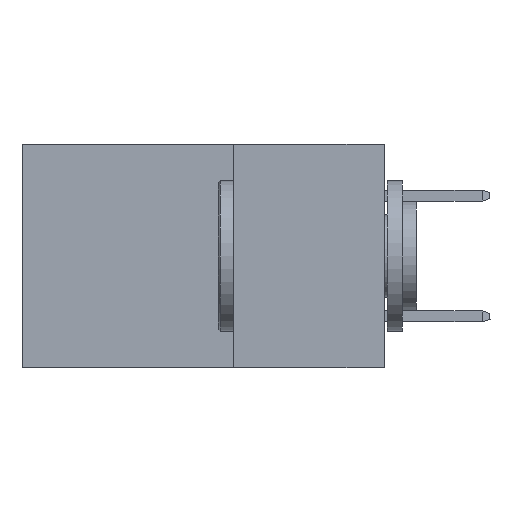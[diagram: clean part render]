
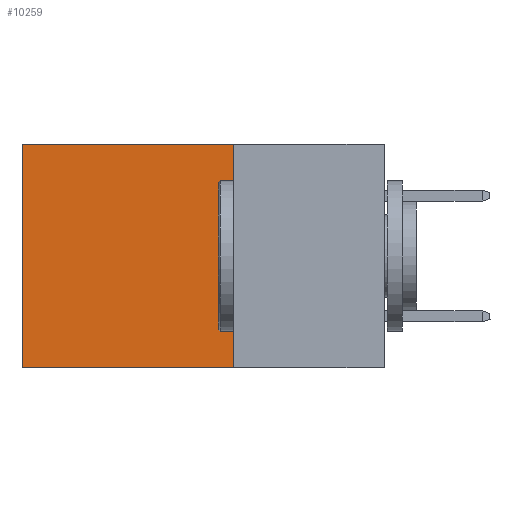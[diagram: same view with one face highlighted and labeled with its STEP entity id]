
A CAD part, left-side view. The second image highlights one B-rep face of the part: STEP entity #10259.
In plain terms, the highlighted planar face has unit normal (-1, 0, 0).
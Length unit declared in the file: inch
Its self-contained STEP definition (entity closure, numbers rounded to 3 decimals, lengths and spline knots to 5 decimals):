
#1273 = PLANE ( 'NONE',  #4057 ) ;
#2223 = EDGE_CURVE ( 'NONE', #16930, #2907, #3353, .T. ) ;
#2907 = VERTEX_POINT ( 'NONE', #20863 ) ;
#3353 = LINE ( 'NONE', #8130, #25285 ) ;
#3483 = DIRECTION ( 'NONE',  ( 1., 0., 0. ) ) ;
#3954 = DIRECTION ( 'NONE',  ( 0., 1., 0. ) ) ;
#4057 = AXIS2_PLACEMENT_3D ( 'NONE', #14496, #3483, #18888 ) ;
#4997 = ORIENTED_EDGE ( 'NONE', *, *, #21339, .T. ) ;
#5509 = CARTESIAN_POINT ( 'NONE',  ( 0.2615, 0.25, 0. ) ) ;
#6260 = ORIENTED_EDGE ( 'NONE', *, *, #23093, .T. ) ;
#7319 = VECTOR ( 'NONE', #24124, 39.37008 ) ;
#7760 = DIRECTION ( 'NONE',  ( 0., 0., -1. ) ) ;
#8130 = CARTESIAN_POINT ( 'NONE',  ( 0.2615, 0.25, -0.37 ) ) ;
#8234 = ORIENTED_EDGE ( 'NONE', *, *, #2223, .F. ) ;
#9297 = CARTESIAN_POINT ( 'NONE',  ( 0.2615, 0.6, -0.37 ) ) ;
#10007 = CARTESIAN_POINT ( 'NONE',  ( 0.2615, 0.6, 0. ) ) ;
#10259 = ADVANCED_FACE ( 'NONE', ( #20983 ), #1273, .F. ) ;
#11498 = VERTEX_POINT ( 'NONE', #10007 ) ;
#12403 = VECTOR ( 'NONE', #3954, 39.37008 ) ;
#13103 = LINE ( 'NONE', #21358, #12403 ) ;
#13170 = LINE ( 'NONE', #21960, #7319 ) ;
#14496 = CARTESIAN_POINT ( 'NONE',  ( 0.2615, 0.25, -0.37 ) ) ;
#16076 = EDGE_LOOP ( 'NONE', ( #4997, #19718, #8234, #6260 ) ) ;
#16077 = EDGE_CURVE ( 'NONE', #2907, #27691, #13103, .T. ) ;
#16930 = VERTEX_POINT ( 'NONE', #5509 ) ;
#17886 = VECTOR ( 'NONE', #20310, 39.37008 ) ;
#18583 = LINE ( 'NONE', #26707, #17886 ) ;
#18888 = DIRECTION ( 'NONE',  ( 0., 0., -1. ) ) ;
#19718 = ORIENTED_EDGE ( 'NONE', *, *, #16077, .F. ) ;
#20310 = DIRECTION ( 'NONE',  ( 0., 1., 0. ) ) ;
#20863 = CARTESIAN_POINT ( 'NONE',  ( 0.2615, 0.25, -0.37 ) ) ;
#20983 = FACE_OUTER_BOUND ( 'NONE', #16076, .T. ) ;
#21339 = EDGE_CURVE ( 'NONE', #11498, #27691, #13170, .T. ) ;
#21358 = CARTESIAN_POINT ( 'NONE',  ( 0.2615, 0.25, -0.37 ) ) ;
#21960 = CARTESIAN_POINT ( 'NONE',  ( 0.2615, 0.6, -0.37 ) ) ;
#23093 = EDGE_CURVE ( 'NONE', #16930, #11498, #18583, .T. ) ;
#24124 = DIRECTION ( 'NONE',  ( 0., 0., -1. ) ) ;
#25285 = VECTOR ( 'NONE', #7760, 39.37008 ) ;
#26707 = CARTESIAN_POINT ( 'NONE',  ( 0.2615, 0.25, 0. ) ) ;
#27691 = VERTEX_POINT ( 'NONE', #9297 ) ;
